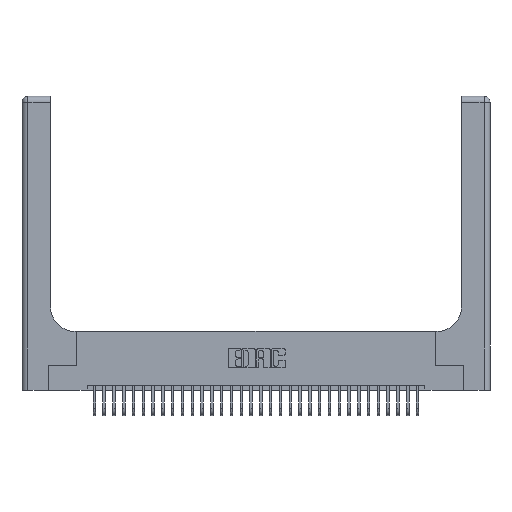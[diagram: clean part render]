
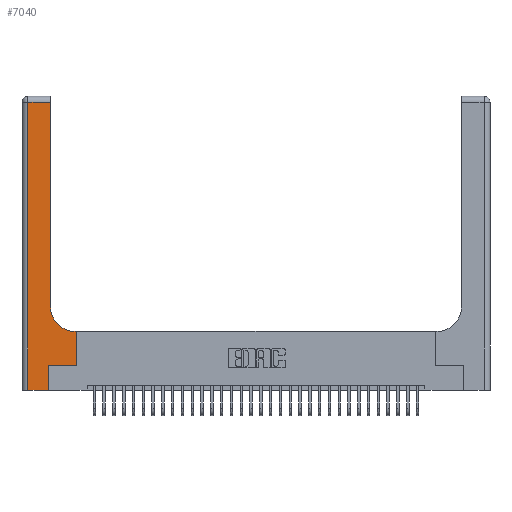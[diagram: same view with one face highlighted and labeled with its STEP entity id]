
A CAD part, top view. The second image highlights one B-rep face of the part: STEP entity #7040.
In plain terms, the highlighted planar face has unit normal (0, 0, 1).
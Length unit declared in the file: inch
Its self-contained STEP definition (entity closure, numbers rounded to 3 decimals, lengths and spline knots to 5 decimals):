
#243 = FACE_OUTER_BOUND ( 'NONE', #13715, .T. ) ;
#813 = LINE ( 'NONE', #29924, #6673 ) ;
#876 = ORIENTED_EDGE ( 'NONE', *, *, #14362, .T. ) ;
#949 = DIRECTION ( 'NONE',  ( 1., 0., 0. ) ) ;
#1151 = ORIENTED_EDGE ( 'NONE', *, *, #20006, .T. ) ;
#1296 = EDGE_CURVE ( 'NONE', #9286, #9045, #2261, .T. ) ;
#1924 = CARTESIAN_POINT ( 'NONE',  ( 0.5415, 0.6, 0.37 ) ) ;
#2261 = LINE ( 'NONE', #15587, #21259 ) ;
#3134 = ORIENTED_EDGE ( 'NONE', *, *, #5179, .T. ) ;
#3225 = ORIENTED_EDGE ( 'NONE', *, *, #11688, .T. ) ;
#3805 = CARTESIAN_POINT ( 'NONE',  ( 0., 3., 0.37 ) ) ;
#4018 = VERTEX_POINT ( 'NONE', #21946 ) ;
#4052 = CIRCLE ( 'NONE', #27699, 0.25 ) ;
#5179 = EDGE_CURVE ( 'NONE', #16481, #9286, #29270, .T. ) ;
#5435 = DIRECTION ( 'NONE',  ( 0., -1., 0. ) ) ;
#6231 = EDGE_CURVE ( 'NONE', #16316, #11611, #24293, .T. ) ;
#6327 = DIRECTION ( 'NONE',  ( 0., 0., -1. ) ) ;
#6673 = VECTOR ( 'NONE', #5435, 39.37008 ) ;
#7040 = ADVANCED_FACE ( 'NONE', ( #243 ), #30802, .F. ) ;
#7729 = VERTEX_POINT ( 'NONE', #31168 ) ;
#7771 = AXIS2_PLACEMENT_3D ( 'NONE', #3805, #6327, #23551 ) ;
#8510 = CARTESIAN_POINT ( 'NONE',  ( 0.269, 0.25, 0.37 ) ) ;
#8566 = ORIENTED_EDGE ( 'NONE', *, *, #19113, .T. ) ;
#8955 = EDGE_CURVE ( 'NONE', #4018, #18631, #31349, .T. ) ;
#9045 = VERTEX_POINT ( 'NONE', #1924 ) ;
#9286 = VERTEX_POINT ( 'NONE', #24910 ) ;
#10928 = CARTESIAN_POINT ( 'NONE',  ( 0.5585, 0.25, 0.37 ) ) ;
#11611 = VERTEX_POINT ( 'NONE', #14510 ) ;
#11641 = DIRECTION ( 'NONE',  ( 1., 0., 0. ) ) ;
#11688 = EDGE_CURVE ( 'NONE', #18631, #31814, #15445, .T. ) ;
#12002 = DIRECTION ( 'NONE',  ( 0., 1., 0. ) ) ;
#12489 = ORIENTED_EDGE ( 'NONE', *, *, #8955, .T. ) ;
#13108 = DIRECTION ( 'NONE',  ( -1., 0., 0. ) ) ;
#13715 = EDGE_LOOP ( 'NONE', ( #27311, #8566, #25858, #12489, #3225, #1151, #3134, #19439, #876 ) ) ;
#14362 = EDGE_CURVE ( 'NONE', #9045, #16316, #4052, .T. ) ;
#14510 = CARTESIAN_POINT ( 'NONE',  ( 0.2915, 2.94, 0.37 ) ) ;
#15219 = CARTESIAN_POINT ( 'NONE',  ( 0.2915, 0.85, 0.37 ) ) ;
#15445 = LINE ( 'NONE', #24559, #26900 ) ;
#15587 = CARTESIAN_POINT ( 'NONE',  ( 0.2915, 0.6, 0.37 ) ) ;
#15822 = DIRECTION ( 'NONE',  ( 0., 0., -1. ) ) ;
#16316 = VERTEX_POINT ( 'NONE', #15219 ) ;
#16481 = VERTEX_POINT ( 'NONE', #10928 ) ;
#16649 = CARTESIAN_POINT ( 'NONE',  ( 0.2915, 3., 0.37 ) ) ;
#16755 = LINE ( 'NONE', #28359, #28985 ) ;
#17624 = DIRECTION ( 'NONE',  ( -1., 0., 0. ) ) ;
#17794 = VECTOR ( 'NONE', #21505, 39.37008 ) ;
#18404 = VECTOR ( 'NONE', #11641, 39.37008 ) ;
#18631 = VERTEX_POINT ( 'NONE', #20483 ) ;
#19113 = EDGE_CURVE ( 'NONE', #11611, #7729, #29050, .T. ) ;
#19439 = ORIENTED_EDGE ( 'NONE', *, *, #1296, .T. ) ;
#19860 = CARTESIAN_POINT ( 'NONE',  ( 0.5585, 0.25, 0.37 ) ) ;
#20006 = EDGE_CURVE ( 'NONE', #31814, #16481, #16755, .T. ) ;
#20349 = EDGE_CURVE ( 'NONE', #7729, #4018, #813, .T. ) ;
#20483 = CARTESIAN_POINT ( 'NONE',  ( 0.269, 0., 0.37 ) ) ;
#21259 = VECTOR ( 'NONE', #13108, 39.37008 ) ;
#21431 = CARTESIAN_POINT ( 'NONE',  ( 0., 0., 0.37 ) ) ;
#21505 = DIRECTION ( 'NONE',  ( 0., 1., 0. ) ) ;
#21946 = CARTESIAN_POINT ( 'NONE',  ( 0.06, 0., 0.37 ) ) ;
#22574 = VECTOR ( 'NONE', #17624, 39.37008 ) ;
#23549 = VECTOR ( 'NONE', #12002, 39.37008 ) ;
#23551 = DIRECTION ( 'NONE',  ( -1., 0., 0. ) ) ;
#24293 = LINE ( 'NONE', #16649, #17794 ) ;
#24559 = CARTESIAN_POINT ( 'NONE',  ( 0.269, 0., 0.37 ) ) ;
#24910 = CARTESIAN_POINT ( 'NONE',  ( 0.5585, 0.6, 0.37 ) ) ;
#25858 = ORIENTED_EDGE ( 'NONE', *, *, #20349, .T. ) ;
#26900 = VECTOR ( 'NONE', #31892, 39.37008 ) ;
#27311 = ORIENTED_EDGE ( 'NONE', *, *, #6231, .T. ) ;
#27699 = AXIS2_PLACEMENT_3D ( 'NONE', #30463, #15822, #949 ) ;
#28359 = CARTESIAN_POINT ( 'NONE',  ( 0.269, 0.25, 0.37 ) ) ;
#28985 = VECTOR ( 'NONE', #30805, 39.37008 ) ;
#29050 = LINE ( 'NONE', #29791, #22574 ) ;
#29270 = LINE ( 'NONE', #19860, #23549 ) ;
#29791 = CARTESIAN_POINT ( 'NONE',  ( 0., 2.94, 0.37 ) ) ;
#29924 = CARTESIAN_POINT ( 'NONE',  ( 0.06, 3., 0.37 ) ) ;
#30463 = CARTESIAN_POINT ( 'NONE',  ( 0.5415, 0.85, 0.37 ) ) ;
#30802 = PLANE ( 'NONE',  #7771 ) ;
#30805 = DIRECTION ( 'NONE',  ( 1., 0., 0. ) ) ;
#31168 = CARTESIAN_POINT ( 'NONE',  ( 0.06, 2.94, 0.37 ) ) ;
#31349 = LINE ( 'NONE', #21431, #18404 ) ;
#31814 = VERTEX_POINT ( 'NONE', #8510 ) ;
#31892 = DIRECTION ( 'NONE',  ( 0., 1., 0. ) ) ;
